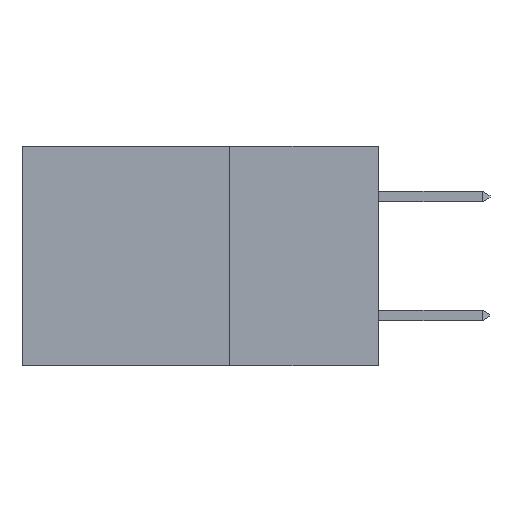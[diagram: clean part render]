
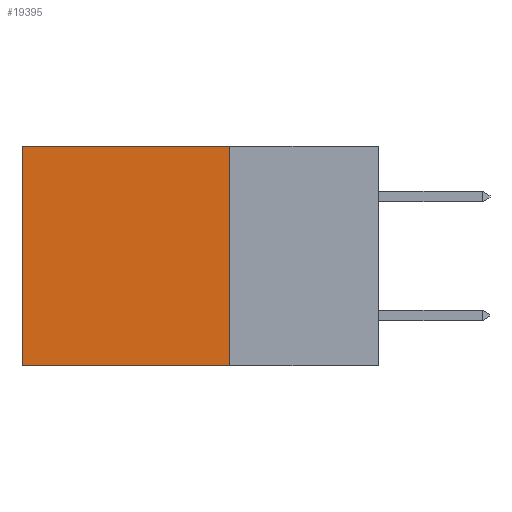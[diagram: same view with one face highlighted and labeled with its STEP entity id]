
A CAD part, left-side view. The second image highlights one B-rep face of the part: STEP entity #19395.
In plain terms, the highlighted planar face has unit normal (-1, 0, 0).
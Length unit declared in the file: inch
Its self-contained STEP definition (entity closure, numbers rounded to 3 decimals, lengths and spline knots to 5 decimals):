
#265 = LINE ( 'NONE', #8849, #24022 ) ;
#1052 = PLANE ( 'NONE',  #11023 ) ;
#1075 = CARTESIAN_POINT ( 'NONE',  ( 0.298, 0.25, 0. ) ) ;
#2249 = EDGE_CURVE ( 'NONE', #20912, #5328, #11647, .T. ) ;
#2255 = VECTOR ( 'NONE', #23823, 39.37008 ) ;
#2409 = ORIENTED_EDGE ( 'NONE', *, *, #2249, .F. ) ;
#2909 = EDGE_CURVE ( 'NONE', #5328, #14697, #7182, .T. ) ;
#3248 = EDGE_LOOP ( 'NONE', ( #13623, #13535, #2409, #5536 ) ) ;
#5328 = VERTEX_POINT ( 'NONE', #14796 ) ;
#5536 = ORIENTED_EDGE ( 'NONE', *, *, #21070, .T. ) ;
#6496 = CARTESIAN_POINT ( 'NONE',  ( 0.298, 0.25, -0.37 ) ) ;
#7182 = LINE ( 'NONE', #6496, #2255 ) ;
#7785 = FACE_OUTER_BOUND ( 'NONE', #3248, .T. ) ;
#8525 = EDGE_CURVE ( 'NONE', #20532, #14697, #265, .T. ) ;
#8584 = CARTESIAN_POINT ( 'NONE',  ( 0.298, 0.25, 0. ) ) ;
#8849 = CARTESIAN_POINT ( 'NONE',  ( 0.298, 0.6, 0. ) ) ;
#9596 = VECTOR ( 'NONE', #11360, 39.37008 ) ;
#10469 = DIRECTION ( 'NONE',  ( 0., 0., -1. ) ) ;
#10748 = DIRECTION ( 'NONE',  ( 0., 0., -1. ) ) ;
#11023 = AXIS2_PLACEMENT_3D ( 'NONE', #8584, #21813, #10469 ) ;
#11045 = VECTOR ( 'NONE', #22706, 39.37008 ) ;
#11360 = DIRECTION ( 'NONE',  ( 0., 1., 0. ) ) ;
#11647 = LINE ( 'NONE', #1075, #11045 ) ;
#13535 = ORIENTED_EDGE ( 'NONE', *, *, #2909, .F. ) ;
#13623 = ORIENTED_EDGE ( 'NONE', *, *, #8525, .T. ) ;
#14697 = VERTEX_POINT ( 'NONE', #17108 ) ;
#14796 = CARTESIAN_POINT ( 'NONE',  ( 0.298, 0.25, -0.37 ) ) ;
#17052 = CARTESIAN_POINT ( 'NONE',  ( 0.298, 0.25, 0. ) ) ;
#17108 = CARTESIAN_POINT ( 'NONE',  ( 0.298, 0.6, -0.37 ) ) ;
#19395 = ADVANCED_FACE ( 'NONE', ( #7785 ), #1052, .F. ) ;
#20237 = CARTESIAN_POINT ( 'NONE',  ( 0.298, 0.25, 0. ) ) ;
#20322 = LINE ( 'NONE', #17052, #9596 ) ;
#20532 = VERTEX_POINT ( 'NONE', #20826 ) ;
#20826 = CARTESIAN_POINT ( 'NONE',  ( 0.298, 0.6, 0. ) ) ;
#20912 = VERTEX_POINT ( 'NONE', #20237 ) ;
#21070 = EDGE_CURVE ( 'NONE', #20912, #20532, #20322, .T. ) ;
#21813 = DIRECTION ( 'NONE',  ( 1., 0., 0. ) ) ;
#22706 = DIRECTION ( 'NONE',  ( 0., 0., -1. ) ) ;
#23823 = DIRECTION ( 'NONE',  ( 0., 1., 0. ) ) ;
#24022 = VECTOR ( 'NONE', #10748, 39.37008 ) ;
